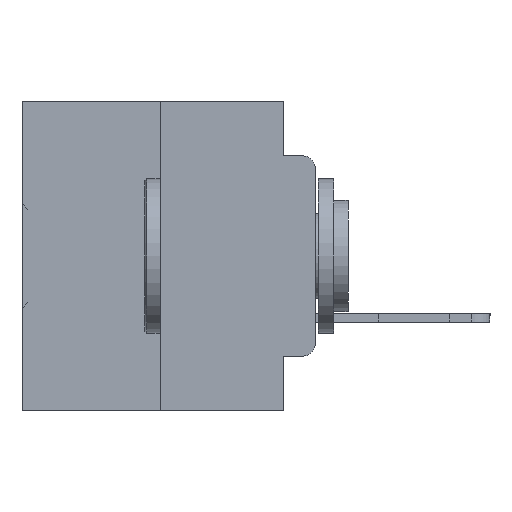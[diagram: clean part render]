
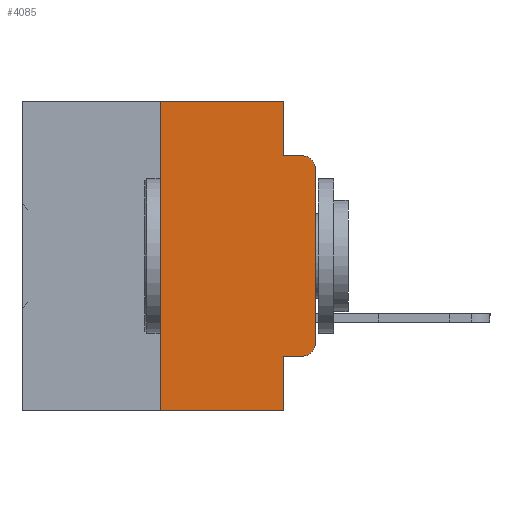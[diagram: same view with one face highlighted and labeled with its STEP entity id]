
A CAD part, left-side view. The second image highlights one B-rep face of the part: STEP entity #4085.
In plain terms, the highlighted planar face has unit normal (-1, 0, 0).
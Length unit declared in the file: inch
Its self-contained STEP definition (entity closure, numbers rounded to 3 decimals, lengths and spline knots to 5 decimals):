
#414 = EDGE_LOOP ( 'NONE', ( #13539, #28286, #1183, #8707, #25240, #26118, #33419, #5497, #4175, #12570 ) ) ;
#853 = DIRECTION ( 'NONE',  ( 0., -1., 0. ) ) ;
#919 = DIRECTION ( 'NONE',  ( 1., 0., 0. ) ) ;
#944 = VERTEX_POINT ( 'NONE', #13757 ) ;
#1183 = ORIENTED_EDGE ( 'NONE', *, *, #16588, .F. ) ;
#1286 = DIRECTION ( 'NONE',  ( -1., 0., 0. ) ) ;
#1756 = CIRCLE ( 'NONE', #10558, 0.02 ) ;
#1895 = VERTEX_POINT ( 'NONE', #10562 ) ;
#2408 = LINE ( 'NONE', #9135, #23830 ) ;
#2474 = VECTOR ( 'NONE', #14179, 39.37008 ) ;
#2512 = DIRECTION ( 'NONE',  ( -1., 0., 0. ) ) ;
#2520 = CARTESIAN_POINT ( 'NONE',  ( 0., 0.051, -0.4115 ) ) ;
#2723 = AXIS2_PLACEMENT_3D ( 'NONE', #19299, #2512, #22074 ) ;
#2873 = LINE ( 'NONE', #34179, #23430 ) ;
#2913 = CARTESIAN_POINT ( 'NONE',  ( 0., 0.051, 0. ) ) ;
#3417 = EDGE_CURVE ( 'NONE', #13696, #3917, #24978, .T. ) ;
#3909 = AXIS2_PLACEMENT_3D ( 'NONE', #34256, #919, #20502 ) ;
#3917 = VERTEX_POINT ( 'NONE', #8593 ) ;
#4085 = ADVANCED_FACE ( 'NONE', ( #33980 ), #14955, .F. ) ;
#4175 = ORIENTED_EDGE ( 'NONE', *, *, #32133, .T. ) ;
#5497 = ORIENTED_EDGE ( 'NONE', *, *, #3417, .F. ) ;
#5578 = LINE ( 'NONE', #34596, #19567 ) ;
#5763 = DIRECTION ( 'NONE',  ( 0., 0., -1. ) ) ;
#6232 = CARTESIAN_POINT ( 'NONE',  ( 0., 0., -0.1085 ) ) ;
#7218 = EDGE_CURVE ( 'NONE', #944, #8510, #5578, .T. ) ;
#7517 = VERTEX_POINT ( 'NONE', #32050 ) ;
#7909 = CARTESIAN_POINT ( 'NONE',  ( 0., 0.473, 0. ) ) ;
#8510 = VERTEX_POINT ( 'NONE', #19868 ) ;
#8593 = CARTESIAN_POINT ( 'NONE',  ( 0., 0.051, -0.5 ) ) ;
#8707 = ORIENTED_EDGE ( 'NONE', *, *, #10991, .F. ) ;
#9135 = CARTESIAN_POINT ( 'NONE',  ( 0., 0., 0. ) ) ;
#9526 = LINE ( 'NONE', #2913, #30810 ) ;
#9730 = VERTEX_POINT ( 'NONE', #6232 ) ;
#9938 = CARTESIAN_POINT ( 'NONE',  ( 0., 0.051, -0.0885 ) ) ;
#10558 = AXIS2_PLACEMENT_3D ( 'NONE', #18096, #1286, #20876 ) ;
#10562 = CARTESIAN_POINT ( 'NONE',  ( 0., 0.02, -0.4115 ) ) ;
#10879 = LINE ( 'NONE', #25193, #2474 ) ;
#10991 = EDGE_CURVE ( 'NONE', #7517, #30142, #9526, .T. ) ;
#11033 = VECTOR ( 'NONE', #19313, 39.37008 ) ;
#11775 = VERTEX_POINT ( 'NONE', #12129 ) ;
#12129 = CARTESIAN_POINT ( 'NONE',  ( 0., 0.02, -0.0885 ) ) ;
#12546 = VECTOR ( 'NONE', #19133, 39.37008 ) ;
#12570 = ORIENTED_EDGE ( 'NONE', *, *, #28445, .T. ) ;
#12638 = DIRECTION ( 'NONE',  ( 0., 0., 1. ) ) ;
#13539 = ORIENTED_EDGE ( 'NONE', *, *, #25869, .T. ) ;
#13696 = VERTEX_POINT ( 'NONE', #18211 ) ;
#13757 = CARTESIAN_POINT ( 'NONE',  ( 0., 0.25, -0.5 ) ) ;
#14179 = DIRECTION ( 'NONE',  ( 0., -1., 0. ) ) ;
#14955 = PLANE ( 'NONE',  #3909 ) ;
#16037 = LINE ( 'NONE', #7909, #12546 ) ;
#16588 = EDGE_CURVE ( 'NONE', #30142, #11775, #2873, .T. ) ;
#17044 = DIRECTION ( 'NONE',  ( 0., 0., -1. ) ) ;
#17618 = VECTOR ( 'NONE', #17044, 39.37008 ) ;
#18096 = CARTESIAN_POINT ( 'NONE',  ( 0., 0.02, -0.1085 ) ) ;
#18211 = CARTESIAN_POINT ( 'NONE',  ( 0., 0.051, -0.4115 ) ) ;
#19133 = DIRECTION ( 'NONE',  ( 0., -1., 0. ) ) ;
#19299 = CARTESIAN_POINT ( 'NONE',  ( 0., 0.02, -0.3915 ) ) ;
#19313 = DIRECTION ( 'NONE',  ( 0., -1., 0. ) ) ;
#19567 = VECTOR ( 'NONE', #12638, 39.37008 ) ;
#19868 = CARTESIAN_POINT ( 'NONE',  ( 0., 0.25, 0. ) ) ;
#20288 = EDGE_CURVE ( 'NONE', #9730, #11775, #1756, .T. ) ;
#20502 = DIRECTION ( 'NONE',  ( 0., 0., -1. ) ) ;
#20876 = DIRECTION ( 'NONE',  ( 0., 0., -1. ) ) ;
#22074 = DIRECTION ( 'NONE',  ( 0., 0., -1. ) ) ;
#22244 = VERTEX_POINT ( 'NONE', #32460 ) ;
#23430 = VECTOR ( 'NONE', #853, 39.37008 ) ;
#23830 = VECTOR ( 'NONE', #25780, 39.37008 ) ;
#24272 = EDGE_CURVE ( 'NONE', #944, #3917, #10879, .T. ) ;
#24978 = LINE ( 'NONE', #28091, #17618 ) ;
#25193 = CARTESIAN_POINT ( 'NONE',  ( 0., 0.473, -0.5 ) ) ;
#25240 = ORIENTED_EDGE ( 'NONE', *, *, #29041, .F. ) ;
#25780 = DIRECTION ( 'NONE',  ( 0., 0., 1. ) ) ;
#25869 = EDGE_CURVE ( 'NONE', #22244, #9730, #2408, .T. ) ;
#26118 = ORIENTED_EDGE ( 'NONE', *, *, #7218, .F. ) ;
#28091 = CARTESIAN_POINT ( 'NONE',  ( 0., 0.051, 0. ) ) ;
#28286 = ORIENTED_EDGE ( 'NONE', *, *, #20288, .T. ) ;
#28445 = EDGE_CURVE ( 'NONE', #1895, #22244, #34405, .T. ) ;
#29041 = EDGE_CURVE ( 'NONE', #8510, #7517, #16037, .T. ) ;
#30142 = VERTEX_POINT ( 'NONE', #9938 ) ;
#30810 = VECTOR ( 'NONE', #5763, 39.37008 ) ;
#32050 = CARTESIAN_POINT ( 'NONE',  ( 0., 0.051, 0. ) ) ;
#32133 = EDGE_CURVE ( 'NONE', #13696, #1895, #32293, .T. ) ;
#32293 = LINE ( 'NONE', #2520, #11033 ) ;
#32460 = CARTESIAN_POINT ( 'NONE',  ( 0., 0., -0.3915 ) ) ;
#33419 = ORIENTED_EDGE ( 'NONE', *, *, #24272, .T. ) ;
#33980 = FACE_OUTER_BOUND ( 'NONE', #414, .T. ) ;
#34179 = CARTESIAN_POINT ( 'NONE',  ( 0., 0.051, -0.0885 ) ) ;
#34256 = CARTESIAN_POINT ( 'NONE',  ( 0., 0.473, 0. ) ) ;
#34405 = CIRCLE ( 'NONE', #2723, 0.02 ) ;
#34596 = CARTESIAN_POINT ( 'NONE',  ( 0., 0.25, 0. ) ) ;
